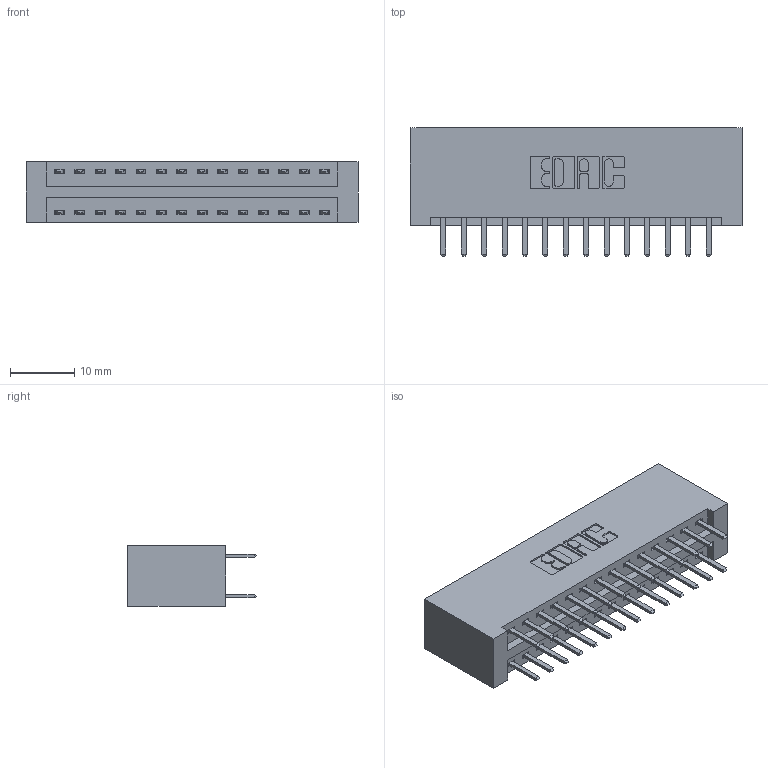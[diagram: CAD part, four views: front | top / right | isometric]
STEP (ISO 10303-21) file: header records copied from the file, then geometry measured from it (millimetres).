
FILE_DESCRIPTION (( 'STEP AP203' ), '1' );
FILE_NAME ('396-028-520-201.STEP', '2018-09-05T02:20:59', ( '' ), ( '' ), 'SwSTEP 2.0', 'SolidWorks 2016', '' );
FILE_SCHEMA (( 'CONFIG_CONTROL_DESIGN' ));
Length unit declared in the file: inch
Products named in the file (3): 396-028-520-201; 346 Part_No Mounting Lugs; 345-292-001_345-293-120
Assembly tree (29 placements, depth 2):
  396-028-520-201
    346 Part_No Mounting Lugs
    345-292-001_345-293-120  x28
Bounding box: 51.69 x 20.02 x 9.4 mm (x, y, z)
Volume: 5383.8 mm3; surface area: 7094.7 mm2
Topology: 29 solids, 29 shells, 1682 faces, 4869 edges, 3170 vertices
Faces by surface type: plane 1108, cylinder 574
Entity records: 12743 total; most frequent: CARTESIAN_POINT 2148, ORIENTED_EDGE 2070, DIRECTION 1927, EDGE_CURVE 1035, VECTOR 851, LINE 851, VERTEX_POINT 686, AXIS2_PLACEMENT_3D 538
